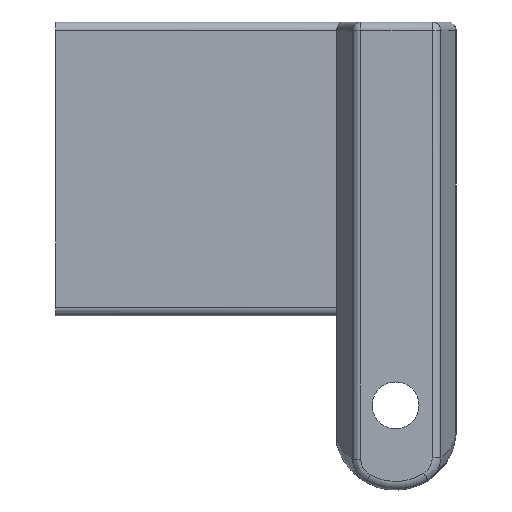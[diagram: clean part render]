
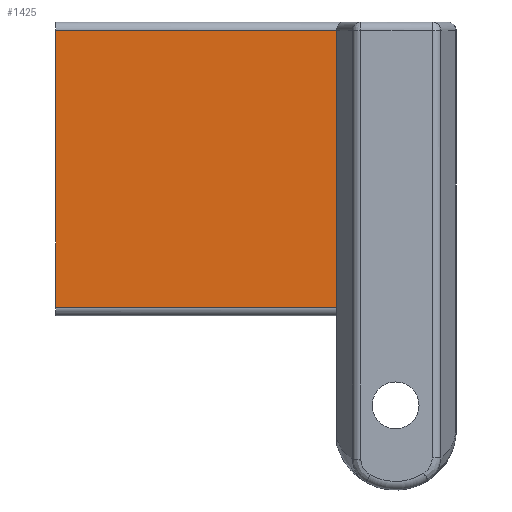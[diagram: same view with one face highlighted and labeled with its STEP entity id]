
A CAD part, front view. The second image highlights one B-rep face of the part: STEP entity #1425.
In plain terms, the highlighted planar face has unit normal (0, -1, 0).
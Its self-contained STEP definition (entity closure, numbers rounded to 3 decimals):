
#34 = LINE ( 'NONE', #1088, #355 ) ;
#40 = CARTESIAN_POINT ( 'NONE',  ( -220.21, 17.562, -17.057 ) ) ;
#41 = EDGE_CURVE ( 'NONE', #813, #689, #505, .T. ) ;
#69 = CARTESIAN_POINT ( 'NONE',  ( -218.689, 17.562, 15.503 ) ) ;
#82 = CARTESIAN_POINT ( 'NONE',  ( -252.316, 17.562, -16.057 ) ) ;
#109 = ORIENTED_EDGE ( 'NONE', *, *, #312, .F. ) ;
#110 = ORIENTED_EDGE ( 'NONE', *, *, #1278, .F. ) ;
#115 = CARTESIAN_POINT ( 'NONE',  ( -224.381, 17.562, -5.772 ) ) ;
#120 = LINE ( 'NONE', #69, #773 ) ;
#147 = ORIENTED_EDGE ( 'NONE', *, *, #41, .F. ) ;
#161 = EDGE_CURVE ( 'NONE', #1382, #844, #120, .T. ) ;
#231 = VECTOR ( 'NONE', #960, 1000. ) ;
#244 = FACE_OUTER_BOUND ( 'NONE', #1228, .T. ) ;
#278 = CARTESIAN_POINT ( 'NONE',  ( -220.205, 17.562, 15.503 ) ) ;
#312 = EDGE_CURVE ( 'NONE', #844, #1116, #1222, .T. ) ;
#322 = VECTOR ( 'NONE', #901, 1000. ) ;
#324 = CARTESIAN_POINT ( 'NONE',  ( -252.316, 17.562, -3.025 ) ) ;
#355 = VECTOR ( 'NONE', #403, 1000. ) ;
#403 = DIRECTION ( 'NONE',  ( -1., 0., 0. ) ) ;
#463 = DIRECTION ( 'NONE',  ( 1., 0., 0. ) ) ;
#474 = AXIS2_PLACEMENT_3D ( 'NONE', #115, #1016, #463 ) ;
#505 = LINE ( 'NONE', #975, #231 ) ;
#563 = ORIENTED_EDGE ( 'NONE', *, *, #1198, .T. ) ;
#577 = PLANE ( 'NONE',  #474 ) ;
#659 = EDGE_CURVE ( 'NONE', #1382, #1065, #928, .T. ) ;
#689 = VERTEX_POINT ( 'NONE', #822 ) ;
#697 = CARTESIAN_POINT ( 'NONE',  ( -220.205, 17.562, -4.432 ) ) ;
#762 = CARTESIAN_POINT ( 'NONE',  ( -227.401, 17.562, -17.057 ) ) ;
#764 = ORIENTED_EDGE ( 'NONE', *, *, #161, .F. ) ;
#773 = VECTOR ( 'NONE', #871, 1000. ) ;
#785 = CARTESIAN_POINT ( 'NONE',  ( -252.316, 17.562, 15.503 ) ) ;
#813 = VERTEX_POINT ( 'NONE', #40 ) ;
#822 = CARTESIAN_POINT ( 'NONE',  ( -220.21, 17.562, -16.057 ) ) ;
#844 = VERTEX_POINT ( 'NONE', #278 ) ;
#857 = DIRECTION ( 'NONE',  ( 1., 0., 0. ) ) ;
#871 = DIRECTION ( 'NONE',  ( 1., 0., 0. ) ) ;
#901 = DIRECTION ( 'NONE',  ( 0., 0., -1. ) ) ;
#926 = VECTOR ( 'NONE', #857, 1000. ) ;
#928 = LINE ( 'NONE', #324, #322 ) ;
#960 = DIRECTION ( 'NONE',  ( 0., 0., 1. ) ) ;
#966 = LINE ( 'NONE', #762, #926 ) ;
#975 = CARTESIAN_POINT ( 'NONE',  ( -220.21, 17.562, -8.363 ) ) ;
#1016 = DIRECTION ( 'NONE',  ( 0., -1., 0. ) ) ;
#1065 = VERTEX_POINT ( 'NONE', #82 ) ;
#1088 = CARTESIAN_POINT ( 'NONE',  ( -227.401, 17.562, -16.057 ) ) ;
#1099 = VECTOR ( 'NONE', #1158, 1000. ) ;
#1116 = VERTEX_POINT ( 'NONE', #1291 ) ;
#1158 = DIRECTION ( 'NONE',  ( 0., 0., -1. ) ) ;
#1198 = EDGE_CURVE ( 'NONE', #813, #1116, #966, .T. ) ;
#1222 = LINE ( 'NONE', #697, #1099 ) ;
#1228 = EDGE_LOOP ( 'NONE', ( #1477, #110, #147, #563, #109, #764 ) ) ;
#1278 = EDGE_CURVE ( 'NONE', #689, #1065, #34, .T. ) ;
#1291 = CARTESIAN_POINT ( 'NONE',  ( -220.205, 17.562, -17.057 ) ) ;
#1382 = VERTEX_POINT ( 'NONE', #785 ) ;
#1425 = ADVANCED_FACE ( 'NONE', ( #244 ), #577, .T. ) ;
#1477 = ORIENTED_EDGE ( 'NONE', *, *, #659, .T. ) ;
